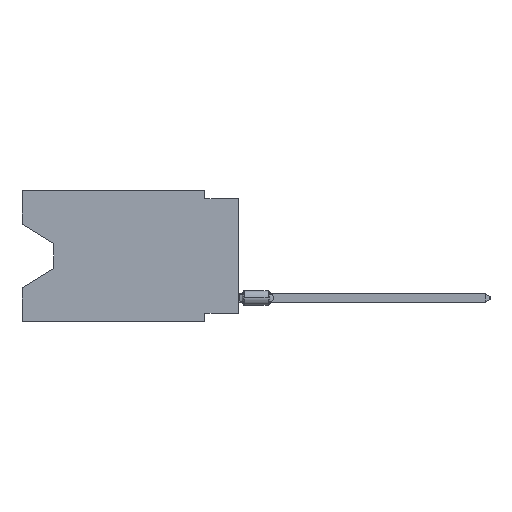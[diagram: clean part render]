
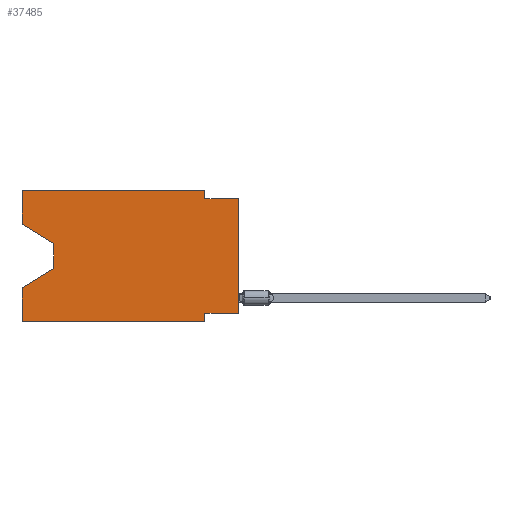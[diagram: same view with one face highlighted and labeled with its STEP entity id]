
A CAD part, left-side view. The second image highlights one B-rep face of the part: STEP entity #37485.
In plain terms, the highlighted planar face has unit normal (-1, 0, 0).
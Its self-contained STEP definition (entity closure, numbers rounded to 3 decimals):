
#24 = CARTESIAN_POINT ( 'NONE',  ( 0., 2.54, -9.906 ) ) ;
#802 = ORIENTED_EDGE ( 'NONE', *, *, #5003, .T. ) ;
#1778 = VERTEX_POINT ( 'NONE', #69443 ) ;
#3088 = EDGE_CURVE ( 'NONE', #42592, #37807, #35472, .T. ) ;
#3581 = CARTESIAN_POINT ( 'NONE',  ( 0., 16.383, -9.906 ) ) ;
#4415 = VERTEX_POINT ( 'NONE', #26569 ) ;
#4516 = DIRECTION ( 'NONE',  ( 0., 0., -1. ) ) ;
#4683 = DIRECTION ( 'NONE',  ( 0., 0., -1. ) ) ;
#5003 = EDGE_CURVE ( 'NONE', #44964, #4415, #7588, .T. ) ;
#5859 = ORIENTED_EDGE ( 'NONE', *, *, #42480, .T. ) ;
#5928 = ORIENTED_EDGE ( 'NONE', *, *, #40212, .F. ) ;
#6637 = EDGE_CURVE ( 'NONE', #17464, #25323, #70192, .T. ) ;
#7458 = CARTESIAN_POINT ( 'NONE',  ( 0., 16.383, 0. ) ) ;
#7588 = LINE ( 'NONE', #69302, #53261 ) ;
#7754 = CARTESIAN_POINT ( 'NONE',  ( 0., 16.383, 0. ) ) ;
#7829 = DIRECTION ( 'NONE',  ( 0., 0.855, -0.519 ) ) ;
#7993 = CARTESIAN_POINT ( 'NONE',  ( 0., 2.54, -9.906 ) ) ;
#8241 = VERTEX_POINT ( 'NONE', #24 ) ;
#9248 = EDGE_CURVE ( 'NONE', #44964, #62804, #18496, .T. ) ;
#10644 = VERTEX_POINT ( 'NONE', #36001 ) ;
#13117 = DIRECTION ( 'NONE',  ( 0., 0., 1. ) ) ;
#13455 = LINE ( 'NONE', #24903, #53396 ) ;
#14324 = CARTESIAN_POINT ( 'NONE',  ( 0., 16.383, -9.906 ) ) ;
#14771 = VECTOR ( 'NONE', #36206, 1000. ) ;
#16047 = CARTESIAN_POINT ( 'NONE',  ( 0., 2.54, -9.271 ) ) ;
#17464 = VERTEX_POINT ( 'NONE', #14324 ) ;
#18496 = LINE ( 'NONE', #41019, #43098 ) ;
#18595 = ORIENTED_EDGE ( 'NONE', *, *, #3088, .T. ) ;
#19695 = VECTOR ( 'NONE', #7829, 1000. ) ;
#19882 = EDGE_CURVE ( 'NONE', #42592, #1778, #47345, .T. ) ;
#20277 = CARTESIAN_POINT ( 'NONE',  ( 0., 16.383, 0. ) ) ;
#20605 = ORIENTED_EDGE ( 'NONE', *, *, #59016, .T. ) ;
#21089 = DIRECTION ( 'NONE',  ( 0., 0., -1. ) ) ;
#21540 = ORIENTED_EDGE ( 'NONE', *, *, #35859, .F. ) ;
#22240 = DIRECTION ( 'NONE',  ( 1., 0., 0. ) ) ;
#24903 = CARTESIAN_POINT ( 'NONE',  ( 0., 0., -0.635 ) ) ;
#25323 = VERTEX_POINT ( 'NONE', #37422 ) ;
#25448 = ORIENTED_EDGE ( 'NONE', *, *, #19882, .F. ) ;
#26569 = CARTESIAN_POINT ( 'NONE',  ( 0., 0., -0.635 ) ) ;
#27167 = VERTEX_POINT ( 'NONE', #28424 ) ;
#28424 = CARTESIAN_POINT ( 'NONE',  ( 0., 13.97, -5.893 ) ) ;
#28672 = ORIENTED_EDGE ( 'NONE', *, *, #66378, .F. ) ;
#29913 = VECTOR ( 'NONE', #21089, 1000. ) ;
#31065 = LINE ( 'NONE', #47692, #19695 ) ;
#32222 = CARTESIAN_POINT ( 'NONE',  ( 0., 16.383, 0. ) ) ;
#32317 = VECTOR ( 'NONE', #4516, 1000. ) ;
#32432 = AXIS2_PLACEMENT_3D ( 'NONE', #32222, #22240, #66572 ) ;
#33255 = LINE ( 'NONE', #71318, #29913 ) ;
#33693 = ORIENTED_EDGE ( 'NONE', *, *, #9248, .F. ) ;
#34839 = DIRECTION ( 'NONE',  ( 0., 0., 1. ) ) ;
#35472 = LINE ( 'NONE', #36895, #65428 ) ;
#35859 = EDGE_CURVE ( 'NONE', #61698, #10644, #33255, .T. ) ;
#36001 = CARTESIAN_POINT ( 'NONE',  ( 0., 2.54, -0.635 ) ) ;
#36206 = DIRECTION ( 'NONE',  ( 0., -1., 0. ) ) ;
#36393 = EDGE_CURVE ( 'NONE', #62804, #8241, #58195, .T. ) ;
#36886 = LINE ( 'NONE', #7754, #14771 ) ;
#36895 = CARTESIAN_POINT ( 'NONE',  ( 0., 16.383, -2.546 ) ) ;
#37422 = CARTESIAN_POINT ( 'NONE',  ( 0., 16.383, -7.36 ) ) ;
#37485 = ADVANCED_FACE ( 'NONE', ( #60655 ), #61748, .F. ) ;
#37807 = VERTEX_POINT ( 'NONE', #53949 ) ;
#40212 = EDGE_CURVE ( 'NONE', #10644, #4415, #13455, .T. ) ;
#41019 = CARTESIAN_POINT ( 'NONE',  ( 0., 0., -9.271 ) ) ;
#42440 = DIRECTION ( 'NONE',  ( 0., -0.855, -0.519 ) ) ;
#42480 = EDGE_CURVE ( 'NONE', #27167, #25323, #31065, .T. ) ;
#42592 = VERTEX_POINT ( 'NONE', #49147 ) ;
#43098 = VECTOR ( 'NONE', #63553, 1000. ) ;
#44293 = VECTOR ( 'NONE', #4683, 1000. ) ;
#44964 = VERTEX_POINT ( 'NONE', #61724 ) ;
#47072 = VECTOR ( 'NONE', #34839, 1000. ) ;
#47345 = LINE ( 'NONE', #7458, #47072 ) ;
#47692 = CARTESIAN_POINT ( 'NONE',  ( 0., 13.97, -5.893 ) ) ;
#48099 = ORIENTED_EDGE ( 'NONE', *, *, #68558, .T. ) ;
#48416 = EDGE_LOOP ( 'NONE', ( #18595, #48099, #5859, #71754, #20605, #64013, #33693, #802, #5928, #21540, #28672, #25448 ) ) ;
#49147 = CARTESIAN_POINT ( 'NONE',  ( 0., 16.383, -2.546 ) ) ;
#52827 = DIRECTION ( 'NONE',  ( 0., 0., 1. ) ) ;
#53261 = VECTOR ( 'NONE', #13117, 1000. ) ;
#53323 = DIRECTION ( 'NONE',  ( 0., -1., 0. ) ) ;
#53396 = VECTOR ( 'NONE', #53323, 1000. ) ;
#53949 = CARTESIAN_POINT ( 'NONE',  ( 0., 13.97, -4.013 ) ) ;
#55279 = CARTESIAN_POINT ( 'NONE',  ( 0., 13.97, -4.013 ) ) ;
#55631 = LINE ( 'NONE', #55279, #44293 ) ;
#58195 = LINE ( 'NONE', #7993, #32317 ) ;
#59016 = EDGE_CURVE ( 'NONE', #17464, #8241, #60837, .T. ) ;
#60655 = FACE_OUTER_BOUND ( 'NONE', #48416, .T. ) ;
#60837 = LINE ( 'NONE', #3581, #69144 ) ;
#61199 = DIRECTION ( 'NONE',  ( 0., -1., 0. ) ) ;
#61698 = VERTEX_POINT ( 'NONE', #63652 ) ;
#61724 = CARTESIAN_POINT ( 'NONE',  ( 0., 0., -9.271 ) ) ;
#61748 = PLANE ( 'NONE',  #32432 ) ;
#62804 = VERTEX_POINT ( 'NONE', #16047 ) ;
#63553 = DIRECTION ( 'NONE',  ( 0., 1., 0. ) ) ;
#63652 = CARTESIAN_POINT ( 'NONE',  ( 0., 2.54, 0. ) ) ;
#64013 = ORIENTED_EDGE ( 'NONE', *, *, #36393, .F. ) ;
#65428 = VECTOR ( 'NONE', #42440, 1000. ) ;
#66378 = EDGE_CURVE ( 'NONE', #1778, #61698, #36886, .T. ) ;
#66572 = DIRECTION ( 'NONE',  ( 0., 0., -1. ) ) ;
#68558 = EDGE_CURVE ( 'NONE', #37807, #27167, #55631, .T. ) ;
#68998 = VECTOR ( 'NONE', #52827, 1000. ) ;
#69144 = VECTOR ( 'NONE', #61199, 1000. ) ;
#69302 = CARTESIAN_POINT ( 'NONE',  ( 0., 0., 0. ) ) ;
#69443 = CARTESIAN_POINT ( 'NONE',  ( 0., 16.383, 0. ) ) ;
#70192 = LINE ( 'NONE', #20277, #68998 ) ;
#71318 = CARTESIAN_POINT ( 'NONE',  ( 0., 2.54, 0. ) ) ;
#71754 = ORIENTED_EDGE ( 'NONE', *, *, #6637, .F. ) ;
